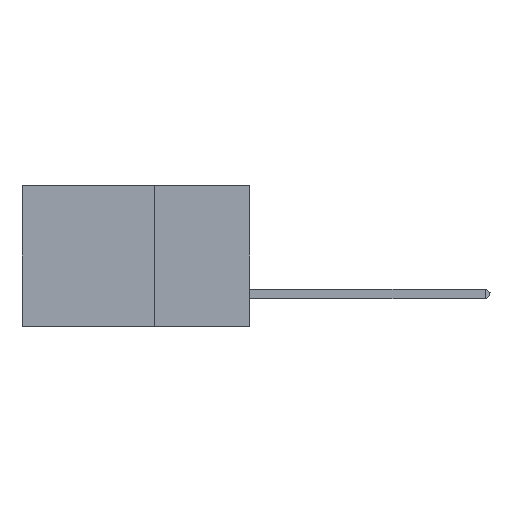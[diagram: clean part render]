
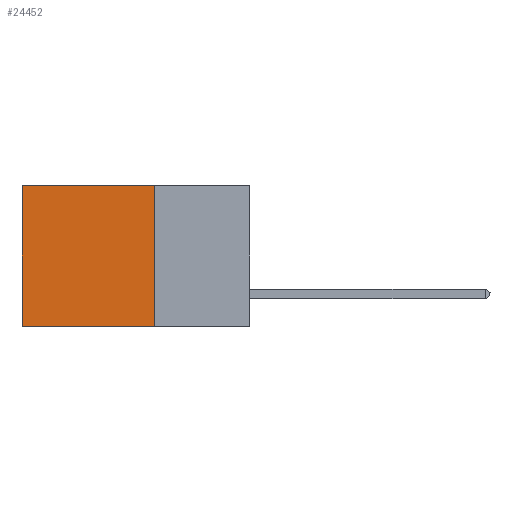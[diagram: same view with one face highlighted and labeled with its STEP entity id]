
A CAD part, left-side view. The second image highlights one B-rep face of the part: STEP entity #24452.
In plain terms, the highlighted planar face has unit normal (-1, 0, 0).
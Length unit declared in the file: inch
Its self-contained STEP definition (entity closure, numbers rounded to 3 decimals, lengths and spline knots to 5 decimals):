
#465 = LINE ( 'NONE', #1800, #8645 ) ;
#1650 = DIRECTION ( 'NONE',  ( 1., 0., 0. ) ) ;
#1751 = EDGE_LOOP ( 'NONE', ( #13328, #19322, #22916, #8025 ) ) ;
#1800 = CARTESIAN_POINT ( 'NONE',  ( 0.2875, 0.25, 0. ) ) ;
#2488 = VERTEX_POINT ( 'NONE', #27235 ) ;
#5298 = EDGE_CURVE ( 'NONE', #7612, #31476, #10702, .T. ) ;
#6371 = EDGE_CURVE ( 'NONE', #19966, #2488, #465, .T. ) ;
#7612 = VERTEX_POINT ( 'NONE', #23773 ) ;
#8025 = ORIENTED_EDGE ( 'NONE', *, *, #6371, .T. ) ;
#8645 = VECTOR ( 'NONE', #38967, 39.37008 ) ;
#9832 = FACE_OUTER_BOUND ( 'NONE', #1751, .T. ) ;
#9985 = VECTOR ( 'NONE', #36403, 39.37008 ) ;
#10702 = LINE ( 'NONE', #23002, #37452 ) ;
#13328 = ORIENTED_EDGE ( 'NONE', *, *, #22803, .T. ) ;
#13822 = CARTESIAN_POINT ( 'NONE',  ( 0.2875, 0.25, 0. ) ) ;
#15227 = CARTESIAN_POINT ( 'NONE',  ( 0.2875, 0.6, 0. ) ) ;
#15531 = CARTESIAN_POINT ( 'NONE',  ( 0.2875, 0.6, -0.37 ) ) ;
#19322 = ORIENTED_EDGE ( 'NONE', *, *, #5298, .F. ) ;
#19966 = VERTEX_POINT ( 'NONE', #38372 ) ;
#20379 = DIRECTION ( 'NONE',  ( 0., 0., -1. ) ) ;
#20568 = LINE ( 'NONE', #15227, #9985 ) ;
#22734 = AXIS2_PLACEMENT_3D ( 'NONE', #13822, #1650, #20379 ) ;
#22803 = EDGE_CURVE ( 'NONE', #2488, #31476, #20568, .T. ) ;
#22916 = ORIENTED_EDGE ( 'NONE', *, *, #25859, .F. ) ;
#22940 = DIRECTION ( 'NONE',  ( 0., 0., -1. ) ) ;
#23002 = CARTESIAN_POINT ( 'NONE',  ( 0.2875, 0.25, -0.37 ) ) ;
#23137 = DIRECTION ( 'NONE',  ( 0., 1., 0. ) ) ;
#23773 = CARTESIAN_POINT ( 'NONE',  ( 0.2875, 0.25, -0.37 ) ) ;
#24452 = ADVANCED_FACE ( 'NONE', ( #9832 ), #38164, .F. ) ;
#25859 = EDGE_CURVE ( 'NONE', #19966, #7612, #33816, .T. ) ;
#27235 = CARTESIAN_POINT ( 'NONE',  ( 0.2875, 0.6, 0. ) ) ;
#29530 = VECTOR ( 'NONE', #22940, 39.37008 ) ;
#31476 = VERTEX_POINT ( 'NONE', #15531 ) ;
#32146 = CARTESIAN_POINT ( 'NONE',  ( 0.2875, 0.25, 0. ) ) ;
#33816 = LINE ( 'NONE', #32146, #29530 ) ;
#36403 = DIRECTION ( 'NONE',  ( 0., 0., -1. ) ) ;
#37452 = VECTOR ( 'NONE', #23137, 39.37008 ) ;
#38164 = PLANE ( 'NONE',  #22734 ) ;
#38372 = CARTESIAN_POINT ( 'NONE',  ( 0.2875, 0.25, 0. ) ) ;
#38967 = DIRECTION ( 'NONE',  ( 0., 1., 0. ) ) ;
